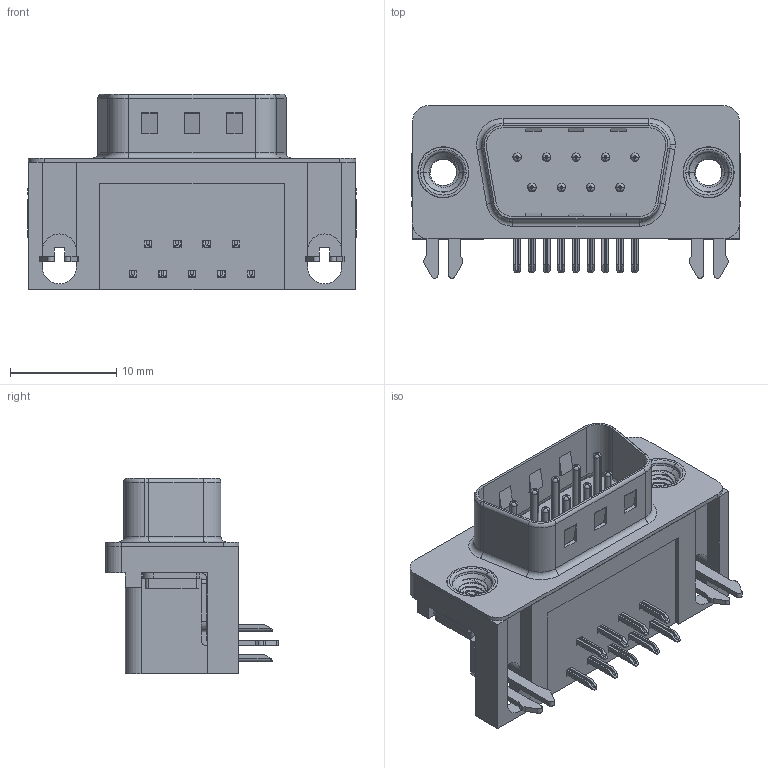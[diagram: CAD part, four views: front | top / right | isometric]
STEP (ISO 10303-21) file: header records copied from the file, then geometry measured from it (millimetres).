
FILE_DESCRIPTION (( 'STEP AP203' ), '1' );
FILE_NAME ('621-009-360-535.STEP', '2019-11-18T20:06:55', ( '' ), ( '' ), 'SwSTEP 2.0', 'SolidWorks 2016', '' );
FILE_SCHEMA (( 'CONFIG_CONTROL_DESIGN' ));
Length unit declared in the file: millimetre
Products named in the file (7): 621 2 Prong Board Lock; 621 Contact Top; 621-009-360-535; 621 Housing_9 Socket; 621 Shell_9 Socket; 621 Contact Bottom; 621 M3 Threaded Rivet
Assembly tree (15 placements, depth 2):
  621-009-360-535
    621 Housing_9 Socket
    621 Shell_9 Socket
    621 Contact Bottom  x4
    621 Contact Top  x5
    621 2 Prong Board Lock  x2
    621 M3 Threaded Rivet  x2
Bounding box: 30.89 x 16.25 x 18.4 mm (x, y, z)
Volume: 3239.8 mm3; surface area: 4429.8 mm2
Topology: 15 solids, 15 shells, 1031 faces, 2603 edges, 1627 vertices
Faces by surface type: plane 605, cylinder 327, torus 85, cone 8, bspline 6
Entity records: 16588 total; most frequent: CARTESIAN_POINT 3918, DIRECTION 2496, ORIENTED_EDGE 2410, EDGE_CURVE 1205, AXIS2_PLACEMENT_3D 851, VECTOR 794, LINE 794, VERTEX_POINT 768
